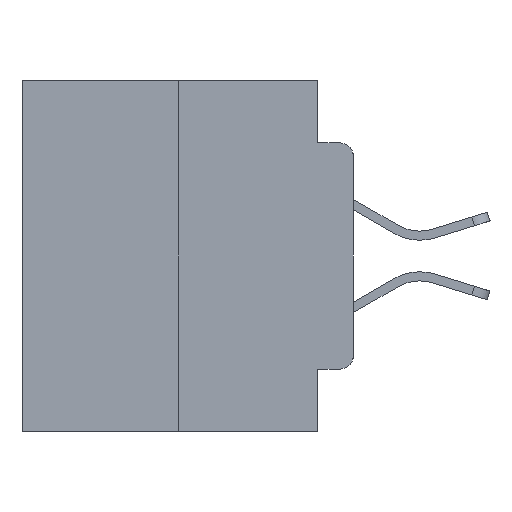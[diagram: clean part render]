
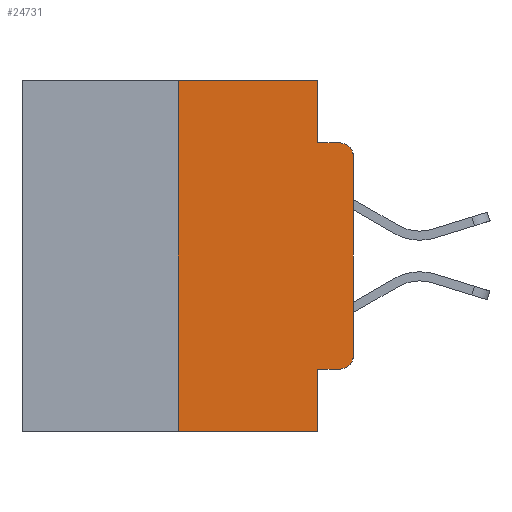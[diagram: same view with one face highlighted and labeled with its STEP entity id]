
A CAD part, left-side view. The second image highlights one B-rep face of the part: STEP entity #24731.
In plain terms, the highlighted planar face has unit normal (-1, 0, 0).
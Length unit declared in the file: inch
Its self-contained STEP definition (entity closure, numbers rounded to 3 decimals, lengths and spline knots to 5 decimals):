
#48 = CARTESIAN_POINT ( 'NONE',  ( 0., 0.051, 0. ) ) ;
#135 = DIRECTION ( 'NONE',  ( 0., -1., 0. ) ) ;
#1242 = DIRECTION ( 'NONE',  ( 0., -1., 0. ) ) ;
#1577 = VERTEX_POINT ( 'NONE', #3276 ) ;
#2132 = VECTOR ( 'NONE', #23607, 39.37008 ) ;
#2303 = EDGE_CURVE ( 'NONE', #2860, #22142, #3781, .T. ) ;
#2860 = VERTEX_POINT ( 'NONE', #25383 ) ;
#2964 = VERTEX_POINT ( 'NONE', #17747 ) ;
#2976 = DIRECTION ( 'NONE',  ( 0., 0., -1. ) ) ;
#3276 = CARTESIAN_POINT ( 'NONE',  ( 0., 0.02, -0.0885 ) ) ;
#3558 = EDGE_CURVE ( 'NONE', #20646, #3719, #4540, .T. ) ;
#3719 = VERTEX_POINT ( 'NONE', #9599 ) ;
#3781 = LINE ( 'NONE', #48, #24702 ) ;
#3882 = CARTESIAN_POINT ( 'NONE',  ( 0., 0.473, 0. ) ) ;
#3993 = VECTOR ( 'NONE', #1242, 39.37008 ) ;
#4320 = CIRCLE ( 'NONE', #11479, 0.02 ) ;
#4540 = LINE ( 'NONE', #19512, #14923 ) ;
#4553 = DIRECTION ( 'NONE',  ( 0., -1., 0. ) ) ;
#5194 = ORIENTED_EDGE ( 'NONE', *, *, #20462, .T. ) ;
#5374 = DIRECTION ( 'NONE',  ( 0., 0., -1. ) ) ;
#5406 = EDGE_CURVE ( 'NONE', #12594, #20646, #6439, .T. ) ;
#5508 = DIRECTION ( 'NONE',  ( 0., -1., 0. ) ) ;
#5651 = CARTESIAN_POINT ( 'NONE',  ( 0., 0., 0. ) ) ;
#6034 = VECTOR ( 'NONE', #4553, 39.37008 ) ;
#6360 = ORIENTED_EDGE ( 'NONE', *, *, #10865, .T. ) ;
#6439 = LINE ( 'NONE', #11646, #2132 ) ;
#6460 = DIRECTION ( 'NONE',  ( -1., 0., 0. ) ) ;
#7083 = DIRECTION ( 'NONE',  ( -1., 0., 0. ) ) ;
#7273 = VECTOR ( 'NONE', #135, 39.37008 ) ;
#7512 = CARTESIAN_POINT ( 'NONE',  ( 0., 0.473, -0.5 ) ) ;
#7701 = VERTEX_POINT ( 'NONE', #13369 ) ;
#8155 = ORIENTED_EDGE ( 'NONE', *, *, #11181, .T. ) ;
#9014 = EDGE_LOOP ( 'NONE', ( #14051, #5194, #15599, #15053, #13357, #12309, #6360, #24376, #8155, #9903 ) ) ;
#9599 = CARTESIAN_POINT ( 'NONE',  ( 0., 0.051, 0. ) ) ;
#9903 = ORIENTED_EDGE ( 'NONE', *, *, #25032, .T. ) ;
#10211 = LINE ( 'NONE', #7512, #3993 ) ;
#10865 = EDGE_CURVE ( 'NONE', #12594, #22142, #10211, .T. ) ;
#10960 = VECTOR ( 'NONE', #2976, 39.37008 ) ;
#11181 = EDGE_CURVE ( 'NONE', #2860, #7701, #23355, .T. ) ;
#11269 = VERTEX_POINT ( 'NONE', #16998 ) ;
#11479 = AXIS2_PLACEMENT_3D ( 'NONE', #18667, #6460, #20640 ) ;
#11646 = CARTESIAN_POINT ( 'NONE',  ( 0., 0.25, 0. ) ) ;
#12135 = FACE_OUTER_BOUND ( 'NONE', #9014, .T. ) ;
#12309 = ORIENTED_EDGE ( 'NONE', *, *, #5406, .F. ) ;
#12594 = VERTEX_POINT ( 'NONE', #25168 ) ;
#13247 = CIRCLE ( 'NONE', #22124, 0.02 ) ;
#13357 = ORIENTED_EDGE ( 'NONE', *, *, #3558, .F. ) ;
#13369 = CARTESIAN_POINT ( 'NONE',  ( 0., 0.02, -0.4115 ) ) ;
#13379 = CARTESIAN_POINT ( 'NONE',  ( 0., 0.051, 0. ) ) ;
#13464 = VERTEX_POINT ( 'NONE', #19171 ) ;
#14051 = ORIENTED_EDGE ( 'NONE', *, *, #22842, .T. ) ;
#14240 = PLANE ( 'NONE',  #17431 ) ;
#14835 = VECTOR ( 'NONE', #17916, 39.37008 ) ;
#14923 = VECTOR ( 'NONE', #5508, 39.37008 ) ;
#15053 = ORIENTED_EDGE ( 'NONE', *, *, #21147, .F. ) ;
#15599 = ORIENTED_EDGE ( 'NONE', *, *, #24314, .F. ) ;
#16363 = LINE ( 'NONE', #13379, #10960 ) ;
#16961 = LINE ( 'NONE', #24798, #6034 ) ;
#16998 = CARTESIAN_POINT ( 'NONE',  ( 0., 0., -0.1085 ) ) ;
#17431 = AXIS2_PLACEMENT_3D ( 'NONE', #3882, #17653, #5374 ) ;
#17653 = DIRECTION ( 'NONE',  ( 1., 0., 0. ) ) ;
#17747 = CARTESIAN_POINT ( 'NONE',  ( 0., 0., -0.3915 ) ) ;
#17916 = DIRECTION ( 'NONE',  ( 0., 0., 1. ) ) ;
#18623 = CARTESIAN_POINT ( 'NONE',  ( 0., 0.051, -0.4115 ) ) ;
#18667 = CARTESIAN_POINT ( 'NONE',  ( 0., 0.02, -0.3915 ) ) ;
#19171 = CARTESIAN_POINT ( 'NONE',  ( 0., 0.051, -0.0885 ) ) ;
#19270 = CARTESIAN_POINT ( 'NONE',  ( 0., 0.02, -0.1085 ) ) ;
#19512 = CARTESIAN_POINT ( 'NONE',  ( 0., 0.473, 0. ) ) ;
#19852 = CARTESIAN_POINT ( 'NONE',  ( 0., 0.25, 0. ) ) ;
#20112 = LINE ( 'NONE', #5651, #14835 ) ;
#20462 = EDGE_CURVE ( 'NONE', #11269, #1577, #13247, .T. ) ;
#20640 = DIRECTION ( 'NONE',  ( 0., 0., -1. ) ) ;
#20646 = VERTEX_POINT ( 'NONE', #19852 ) ;
#21147 = EDGE_CURVE ( 'NONE', #3719, #13464, #16363, .T. ) ;
#21232 = DIRECTION ( 'NONE',  ( 0., 0., -1. ) ) ;
#21635 = CARTESIAN_POINT ( 'NONE',  ( 0., 0.051, -0.5 ) ) ;
#22124 = AXIS2_PLACEMENT_3D ( 'NONE', #19270, #7083, #21232 ) ;
#22142 = VERTEX_POINT ( 'NONE', #21635 ) ;
#22842 = EDGE_CURVE ( 'NONE', #2964, #11269, #20112, .T. ) ;
#23355 = LINE ( 'NONE', #18623, #7273 ) ;
#23383 = DIRECTION ( 'NONE',  ( 0., 0., -1. ) ) ;
#23607 = DIRECTION ( 'NONE',  ( 0., 0., 1. ) ) ;
#24314 = EDGE_CURVE ( 'NONE', #13464, #1577, #16961, .T. ) ;
#24376 = ORIENTED_EDGE ( 'NONE', *, *, #2303, .F. ) ;
#24702 = VECTOR ( 'NONE', #23383, 39.37008 ) ;
#24731 = ADVANCED_FACE ( 'NONE', ( #12135 ), #14240, .F. ) ;
#24798 = CARTESIAN_POINT ( 'NONE',  ( 0., 0.051, -0.0885 ) ) ;
#25032 = EDGE_CURVE ( 'NONE', #7701, #2964, #4320, .T. ) ;
#25168 = CARTESIAN_POINT ( 'NONE',  ( 0., 0.25, -0.5 ) ) ;
#25383 = CARTESIAN_POINT ( 'NONE',  ( 0., 0.051, -0.4115 ) ) ;
